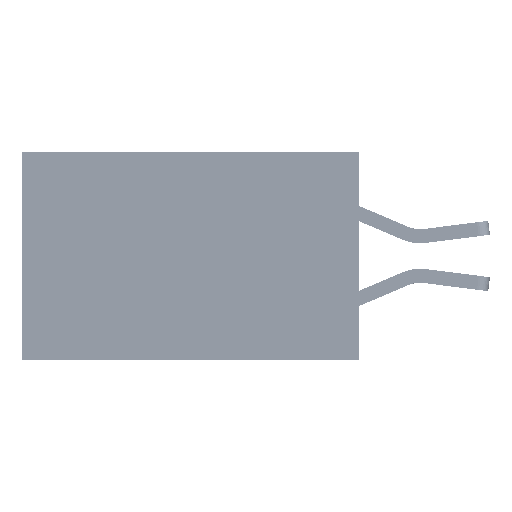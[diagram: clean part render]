
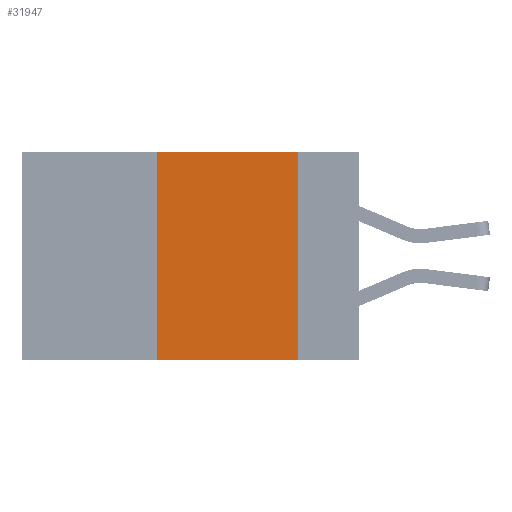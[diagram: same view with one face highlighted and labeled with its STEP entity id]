
A CAD part, left-side view. The second image highlights one B-rep face of the part: STEP entity #31947.
In plain terms, the highlighted planar face has unit normal (-1, 0, 0).
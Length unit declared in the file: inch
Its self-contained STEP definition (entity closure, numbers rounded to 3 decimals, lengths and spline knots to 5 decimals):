
#1310 = ORIENTED_EDGE ( 'NONE', *, *, #31845, .T. ) ;
#6044 = CARTESIAN_POINT ( 'NONE',  ( 0., 0.11, 0. ) ) ;
#8569 = CARTESIAN_POINT ( 'NONE',  ( 0., 0.11, 0. ) ) ;
#12176 = VERTEX_POINT ( 'NONE', #12949 ) ;
#12858 = DIRECTION ( 'NONE',  ( 0., 0., 1. ) ) ;
#12949 = CARTESIAN_POINT ( 'NONE',  ( 0., 0.36, 0. ) ) ;
#14433 = VECTOR ( 'NONE', #35996, 39.37008 ) ;
#15218 = VERTEX_POINT ( 'NONE', #53598 ) ;
#18327 = EDGE_CURVE ( 'NONE', #12176, #19119, #49772, .T. ) ;
#19119 = VERTEX_POINT ( 'NONE', #8569 ) ;
#23514 = CARTESIAN_POINT ( 'NONE',  ( 0., 0.6, -0.37 ) ) ;
#24143 = EDGE_CURVE ( 'NONE', #15218, #12176, #26738, .T. ) ;
#24428 = CARTESIAN_POINT ( 'NONE',  ( 0., 0.6, 0. ) ) ;
#24606 = DIRECTION ( 'NONE',  ( 1., 0., 0. ) ) ;
#26143 = VECTOR ( 'NONE', #52870, 39.37008 ) ;
#26738 = LINE ( 'NONE', #46102, #27353 ) ;
#27353 = VECTOR ( 'NONE', #12858, 39.37008 ) ;
#27438 = ORIENTED_EDGE ( 'NONE', *, *, #37579, .F. ) ;
#29317 = DIRECTION ( 'NONE',  ( 0., 0., -1. ) ) ;
#30040 = FACE_OUTER_BOUND ( 'NONE', #39564, .T. ) ;
#31845 = EDGE_CURVE ( 'NONE', #15218, #38197, #33963, .T. ) ;
#31947 = ADVANCED_FACE ( 'NONE', ( #30040 ), #49731, .F. ) ;
#33922 = AXIS2_PLACEMENT_3D ( 'NONE', #24428, #24606, #29317 ) ;
#33963 = LINE ( 'NONE', #23514, #26143 ) ;
#34564 = DIRECTION ( 'NONE',  ( 0., 0., -1. ) ) ;
#35646 = CARTESIAN_POINT ( 'NONE',  ( 0., 0.6, 0. ) ) ;
#35996 = DIRECTION ( 'NONE',  ( 0., -1., 0. ) ) ;
#37579 = EDGE_CURVE ( 'NONE', #19119, #38197, #46566, .T. ) ;
#38197 = VERTEX_POINT ( 'NONE', #47864 ) ;
#39564 = EDGE_LOOP ( 'NONE', ( #27438, #43473, #39828, #1310 ) ) ;
#39828 = ORIENTED_EDGE ( 'NONE', *, *, #24143, .F. ) ;
#43473 = ORIENTED_EDGE ( 'NONE', *, *, #18327, .F. ) ;
#43972 = VECTOR ( 'NONE', #34564, 39.37008 ) ;
#46102 = CARTESIAN_POINT ( 'NONE',  ( 0., 0.36, 0. ) ) ;
#46566 = LINE ( 'NONE', #6044, #43972 ) ;
#47864 = CARTESIAN_POINT ( 'NONE',  ( 0., 0.11, -0.37 ) ) ;
#49731 = PLANE ( 'NONE',  #33922 ) ;
#49772 = LINE ( 'NONE', #35646, #14433 ) ;
#52870 = DIRECTION ( 'NONE',  ( 0., -1., 0. ) ) ;
#53598 = CARTESIAN_POINT ( 'NONE',  ( 0., 0.36, -0.37 ) ) ;
